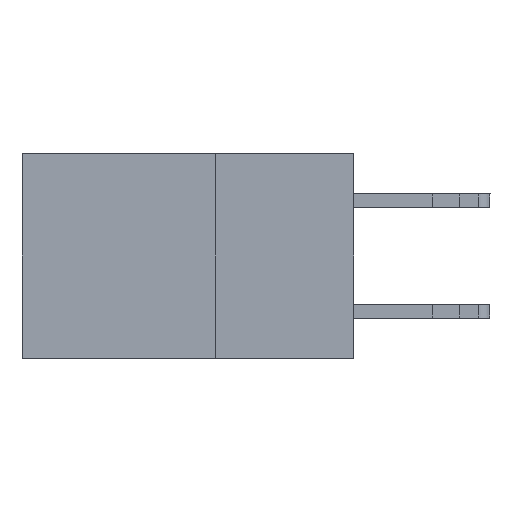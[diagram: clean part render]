
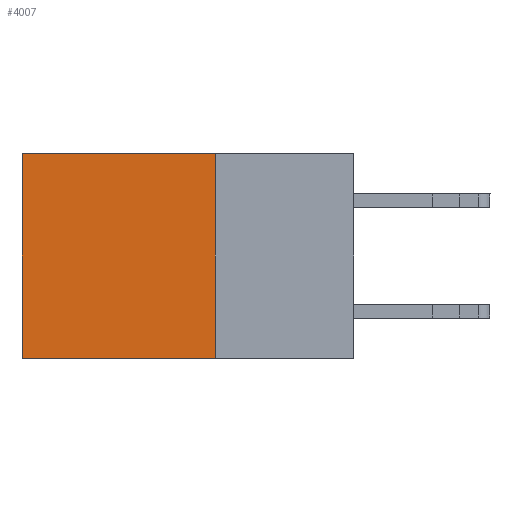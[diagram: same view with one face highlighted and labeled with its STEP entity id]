
A CAD part, left-side view. The second image highlights one B-rep face of the part: STEP entity #4007.
In plain terms, the highlighted planar face has unit normal (-1, 0, 0).
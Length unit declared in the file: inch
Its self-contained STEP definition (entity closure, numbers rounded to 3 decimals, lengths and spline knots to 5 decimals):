
#1094 = EDGE_CURVE ( 'NONE', #34438, #1742, #26401, .T. ) ;
#1487 = ORIENTED_EDGE ( 'NONE', *, *, #24415, .F. ) ;
#1527 = CARTESIAN_POINT ( 'NONE',  ( 0.2875, 0.25, -0.37 ) ) ;
#1724 = VECTOR ( 'NONE', #15575, 39.37008 ) ;
#1742 = VERTEX_POINT ( 'NONE', #2477 ) ;
#2477 = CARTESIAN_POINT ( 'NONE',  ( 0.2875, 0.6, -0.37 ) ) ;
#3930 = DIRECTION ( 'NONE',  ( 0., 0., -1. ) ) ;
#4007 = ADVANCED_FACE ( 'NONE', ( #29621 ), #30569, .F. ) ;
#6161 = VERTEX_POINT ( 'NONE', #34030 ) ;
#6678 = LINE ( 'NONE', #25013, #10573 ) ;
#9090 = DIRECTION ( 'NONE',  ( 1., 0., 0. ) ) ;
#10573 = VECTOR ( 'NONE', #19346, 39.37008 ) ;
#15538 = LINE ( 'NONE', #23086, #1724 ) ;
#15575 = DIRECTION ( 'NONE',  ( 0., 0., -1. ) ) ;
#15997 = VECTOR ( 'NONE', #29506, 39.37008 ) ;
#16294 = CARTESIAN_POINT ( 'NONE',  ( 0.2875, 0.25, -0.37 ) ) ;
#16417 = CARTESIAN_POINT ( 'NONE',  ( 0.2875, 0.6, 0. ) ) ;
#17921 = LINE ( 'NONE', #16294, #15997 ) ;
#18769 = EDGE_CURVE ( 'NONE', #24563, #1742, #17921, .T. ) ;
#19346 = DIRECTION ( 'NONE',  ( 0., 1., 0. ) ) ;
#22753 = CARTESIAN_POINT ( 'NONE',  ( 0.2875, 0.6, 0. ) ) ;
#23086 = CARTESIAN_POINT ( 'NONE',  ( 0.2875, 0.25, 0. ) ) ;
#24415 = EDGE_CURVE ( 'NONE', #6161, #24563, #15538, .T. ) ;
#24563 = VERTEX_POINT ( 'NONE', #1527 ) ;
#25013 = CARTESIAN_POINT ( 'NONE',  ( 0.2875, 0.25, 0. ) ) ;
#26401 = LINE ( 'NONE', #16417, #28276 ) ;
#27093 = ORIENTED_EDGE ( 'NONE', *, *, #18769, .F. ) ;
#28276 = VECTOR ( 'NONE', #3930, 39.37008 ) ;
#29506 = DIRECTION ( 'NONE',  ( 0., 1., 0. ) ) ;
#29621 = FACE_OUTER_BOUND ( 'NONE', #34984, .T. ) ;
#30569 = PLANE ( 'NONE',  #35822 ) ;
#32346 = EDGE_CURVE ( 'NONE', #6161, #34438, #6678, .T. ) ;
#33135 = CARTESIAN_POINT ( 'NONE',  ( 0.2875, 0.25, 0. ) ) ;
#33195 = ORIENTED_EDGE ( 'NONE', *, *, #1094, .T. ) ;
#33908 = ORIENTED_EDGE ( 'NONE', *, *, #32346, .T. ) ;
#34030 = CARTESIAN_POINT ( 'NONE',  ( 0.2875, 0.25, 0. ) ) ;
#34438 = VERTEX_POINT ( 'NONE', #22753 ) ;
#34984 = EDGE_LOOP ( 'NONE', ( #33195, #27093, #1487, #33908 ) ) ;
#35822 = AXIS2_PLACEMENT_3D ( 'NONE', #33135, #9090, #36397 ) ;
#36397 = DIRECTION ( 'NONE',  ( 0., 0., -1. ) ) ;
